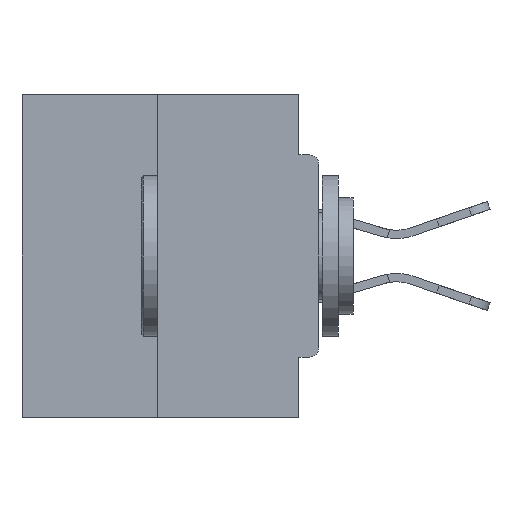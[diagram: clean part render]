
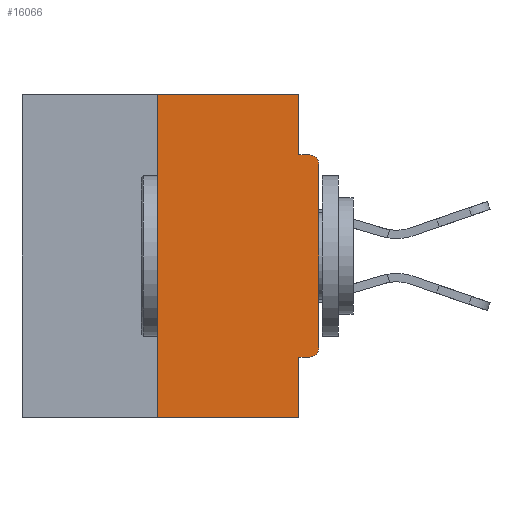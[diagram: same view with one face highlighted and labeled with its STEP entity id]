
A CAD part, left-side view. The second image highlights one B-rep face of the part: STEP entity #16066.
In plain terms, the highlighted planar face has unit normal (-1, 0, 0).
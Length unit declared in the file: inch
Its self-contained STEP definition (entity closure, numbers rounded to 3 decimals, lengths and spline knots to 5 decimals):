
#403 = LINE ( 'NONE', #40973, #18545 ) ;
#769 = ORIENTED_EDGE ( 'NONE', *, *, #25714, .T. ) ;
#1071 = DIRECTION ( 'NONE',  ( 0., 0., -1. ) ) ;
#1255 = LINE ( 'NONE', #16168, #32553 ) ;
#1555 = DIRECTION ( 'NONE',  ( 0., 0., -1. ) ) ;
#2219 = LINE ( 'NONE', #42812, #39766 ) ;
#2297 = CARTESIAN_POINT ( 'NONE',  ( 0., 0., -0.0935 ) ) ;
#3174 = VECTOR ( 'NONE', #30612, 39.37008 ) ;
#3897 = VERTEX_POINT ( 'NONE', #30036 ) ;
#4455 = CARTESIAN_POINT ( 'NONE',  ( 0., 0.031, -0.5 ) ) ;
#4503 = EDGE_CURVE ( 'NONE', #41376, #31161, #41548, .T. ) ;
#5473 = ORIENTED_EDGE ( 'NONE', *, *, #38343, .F. ) ;
#5583 = DIRECTION ( 'NONE',  ( 0., -1., 0. ) ) ;
#6831 = CARTESIAN_POINT ( 'NONE',  ( 0., 0.031, -0.0935 ) ) ;
#8195 = CARTESIAN_POINT ( 'NONE',  ( 0., 0.031, -0.4065 ) ) ;
#8812 = CARTESIAN_POINT ( 'NONE',  ( 0., 0., -0.4065 ) ) ;
#8841 = CARTESIAN_POINT ( 'NONE',  ( 0., 0.25, 0. ) ) ;
#8983 = CARTESIAN_POINT ( 'NONE',  ( 0., 0.015, -0.1085 ) ) ;
#9698 = LINE ( 'NONE', #4455, #23871 ) ;
#9920 = EDGE_CURVE ( 'NONE', #26660, #28977, #1255, .T. ) ;
#10076 = CARTESIAN_POINT ( 'NONE',  ( 0., 0., 0. ) ) ;
#10242 = EDGE_CURVE ( 'NONE', #30589, #10559, #39361, .T. ) ;
#10286 = ORIENTED_EDGE ( 'NONE', *, *, #18938, .F. ) ;
#10559 = VERTEX_POINT ( 'NONE', #21238 ) ;
#11727 = EDGE_CURVE ( 'NONE', #10559, #3897, #33458, .T. ) ;
#12399 = DIRECTION ( 'NONE',  ( -1., 0., 0. ) ) ;
#12678 = CARTESIAN_POINT ( 'NONE',  ( 0., 0.46, 0. ) ) ;
#15454 = FACE_OUTER_BOUND ( 'NONE', #45133, .T. ) ;
#15593 = ORIENTED_EDGE ( 'NONE', *, *, #34787, .F. ) ;
#16035 = VECTOR ( 'NONE', #45448, 39.37008 ) ;
#16066 = ADVANCED_FACE ( 'NONE', ( #15454 ), #21265, .F. ) ;
#16159 = ORIENTED_EDGE ( 'NONE', *, *, #45466, .T. ) ;
#16168 = CARTESIAN_POINT ( 'NONE',  ( 0., 0.25, 0. ) ) ;
#16758 = CARTESIAN_POINT ( 'NONE',  ( 0., 0.031, 0. ) ) ;
#18545 = VECTOR ( 'NONE', #1071, 39.37008 ) ;
#18938 = EDGE_CURVE ( 'NONE', #42673, #39557, #9698, .T. ) ;
#19619 = DIRECTION ( 'NONE',  ( 0., 0., 1. ) ) ;
#21238 = CARTESIAN_POINT ( 'NONE',  ( 0., 0., -0.3915 ) ) ;
#21265 = PLANE ( 'NONE',  #42470 ) ;
#21411 = DIRECTION ( 'NONE',  ( 0., 0., -1. ) ) ;
#22549 = ORIENTED_EDGE ( 'NONE', *, *, #9920, .F. ) ;
#23871 = VECTOR ( 'NONE', #41215, 39.37008 ) ;
#24381 = CARTESIAN_POINT ( 'NONE',  ( 0., 0.015, -0.0935 ) ) ;
#25714 = EDGE_CURVE ( 'NONE', #3897, #31161, #44490, .T. ) ;
#26660 = VERTEX_POINT ( 'NONE', #34691 ) ;
#28117 = ORIENTED_EDGE ( 'NONE', *, *, #10242, .T. ) ;
#28843 = AXIS2_PLACEMENT_3D ( 'NONE', #34207, #12399, #37864 ) ;
#28977 = VERTEX_POINT ( 'NONE', #8841 ) ;
#30036 = CARTESIAN_POINT ( 'NONE',  ( 0., 0., -0.1085 ) ) ;
#30250 = LINE ( 'NONE', #8812, #16035 ) ;
#30589 = VERTEX_POINT ( 'NONE', #34468 ) ;
#30612 = DIRECTION ( 'NONE',  ( 0., -1., 0. ) ) ;
#31161 = VERTEX_POINT ( 'NONE', #24381 ) ;
#31851 = ORIENTED_EDGE ( 'NONE', *, *, #40881, .F. ) ;
#31963 = ORIENTED_EDGE ( 'NONE', *, *, #11727, .T. ) ;
#32467 = DIRECTION ( 'NONE',  ( 1., 0., 0. ) ) ;
#32553 = VECTOR ( 'NONE', #19619, 39.37008 ) ;
#33458 = LINE ( 'NONE', #10076, #35769 ) ;
#33700 = AXIS2_PLACEMENT_3D ( 'NONE', #8983, #37952, #1555 ) ;
#34207 = CARTESIAN_POINT ( 'NONE',  ( 0., 0.015, -0.3915 ) ) ;
#34468 = CARTESIAN_POINT ( 'NONE',  ( 0., 0.015, -0.4065 ) ) ;
#34691 = CARTESIAN_POINT ( 'NONE',  ( 0., 0.25, -0.5 ) ) ;
#34787 = EDGE_CURVE ( 'NONE', #28977, #46712, #41877, .T. ) ;
#35769 = VECTOR ( 'NONE', #46675, 39.37008 ) ;
#37864 = DIRECTION ( 'NONE',  ( 0., 0., -1. ) ) ;
#37952 = DIRECTION ( 'NONE',  ( -1., 0., 0. ) ) ;
#38343 = EDGE_CURVE ( 'NONE', #46712, #41376, #403, .T. ) ;
#39361 = CIRCLE ( 'NONE', #28843, 0.015 ) ;
#39557 = VERTEX_POINT ( 'NONE', #45031 ) ;
#39766 = VECTOR ( 'NONE', #46501, 39.37008 ) ;
#40881 = EDGE_CURVE ( 'NONE', #30589, #42673, #30250, .T. ) ;
#40973 = CARTESIAN_POINT ( 'NONE',  ( 0., 0.031, 0. ) ) ;
#41215 = DIRECTION ( 'NONE',  ( 0., 0., -1. ) ) ;
#41376 = VERTEX_POINT ( 'NONE', #6831 ) ;
#41548 = LINE ( 'NONE', #2297, #46708 ) ;
#41877 = LINE ( 'NONE', #12678, #3174 ) ;
#42470 = AXIS2_PLACEMENT_3D ( 'NONE', #46979, #32467, #21411 ) ;
#42581 = ORIENTED_EDGE ( 'NONE', *, *, #4503, .F. ) ;
#42673 = VERTEX_POINT ( 'NONE', #8195 ) ;
#42812 = CARTESIAN_POINT ( 'NONE',  ( 0., 0.46, -0.5 ) ) ;
#44490 = CIRCLE ( 'NONE', #33700, 0.015 ) ;
#45031 = CARTESIAN_POINT ( 'NONE',  ( 0., 0.031, -0.5 ) ) ;
#45133 = EDGE_LOOP ( 'NONE', ( #15593, #22549, #16159, #10286, #31851, #28117, #31963, #769, #42581, #5473 ) ) ;
#45448 = DIRECTION ( 'NONE',  ( 0., 1., 0. ) ) ;
#45466 = EDGE_CURVE ( 'NONE', #26660, #39557, #2219, .T. ) ;
#46501 = DIRECTION ( 'NONE',  ( 0., -1., 0. ) ) ;
#46675 = DIRECTION ( 'NONE',  ( 0., 0., 1. ) ) ;
#46708 = VECTOR ( 'NONE', #5583, 39.37008 ) ;
#46712 = VERTEX_POINT ( 'NONE', #16758 ) ;
#46979 = CARTESIAN_POINT ( 'NONE',  ( 0., 0.46, 0. ) ) ;
